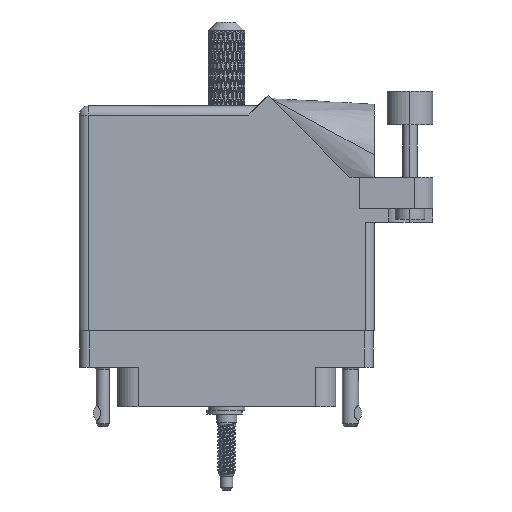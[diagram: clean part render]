
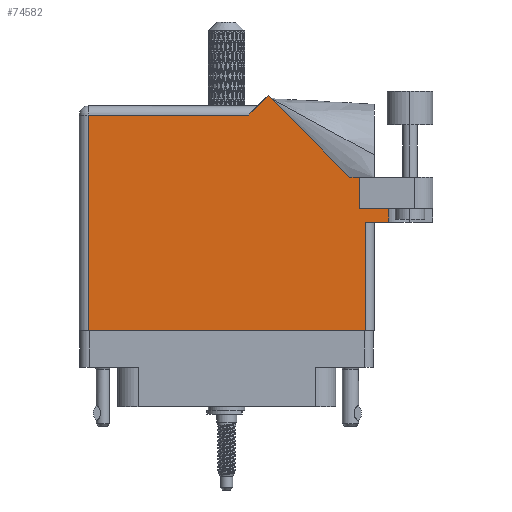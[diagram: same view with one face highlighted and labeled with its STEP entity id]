
A CAD part, front view. The second image highlights one B-rep face of the part: STEP entity #74582.
In plain terms, the highlighted face is planar.
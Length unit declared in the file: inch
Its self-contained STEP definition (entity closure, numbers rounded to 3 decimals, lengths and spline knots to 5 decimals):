
#1 = EDGE_CURVE ( 'NONE', #53166, #113590, #97272, .T. ) ;
#369 = CARTESIAN_POINT ( 'NONE',  ( 0.905, 0.731, 0.455 ) ) ;
#578 = VECTOR ( 'NONE', #109654, 39.37008 ) ;
#999 = DIRECTION ( 'NONE',  ( 0., 1., 0. ) ) ;
#2737 = CARTESIAN_POINT ( 'NONE',  ( 1.1065, 0.731, 0.455 ) ) ;
#3394 = LINE ( 'NONE', #39011, #578 ) ;
#3541 = LINE ( 'NONE', #39164, #83683 ) ;
#3956 = EDGE_CURVE ( 'NONE', #85927, #49844, #56645, .T. ) ;
#6046 = CARTESIAN_POINT ( 'NONE',  ( -1.005, -0.1, 0.455 ) ) ;
#6204 = CARTESIAN_POINT ( 'NONE',  ( 0.83942, 0.944, 0.455 ) ) ;
#7031 = AXIS2_PLACEMENT_3D ( 'NONE', #8806, #87037, #43816 ) ;
#7474 = CARTESIAN_POINT ( 'NONE',  ( -0.943, 1.368, 0.455 ) ) ;
#7632 = CARTESIAN_POINT ( 'NONE',  ( 1.005, 0.637, 0.455 ) ) ;
#8308 = VECTOR ( 'NONE', #999, 39.37008 ) ;
#8493 = DIRECTION ( 'NONE',  ( 0., -1., 0. ) ) ;
#8806 = CARTESIAN_POINT ( 'NONE',  ( -1.005, 1.43, 0.455 ) ) ;
#9829 = CARTESIAN_POINT ( 'NONE',  ( 0.943, -0.1, 0.455 ) ) ;
#13286 = VECTOR ( 'NONE', #91300, 39.37008 ) ;
#14071 = VECTOR ( 'NONE', #58591, 39.37008 ) ;
#14183 = VERTEX_POINT ( 'NONE', #82606 ) ;
#14807 = ORIENTED_EDGE ( 'NONE', *, *, #91940, .T. ) ;
#15362 = VECTOR ( 'NONE', #75333, 39.37008 ) ;
#15830 = CARTESIAN_POINT ( 'NONE',  ( 0.212, 1.43, 0.455 ) ) ;
#16386 = ORIENTED_EDGE ( 'NONE', *, *, #100839, .T. ) ;
#16404 = DIRECTION ( 'NONE',  ( 1., 0., 0. ) ) ;
#17437 = EDGE_CURVE ( 'NONE', #114909, #61215, #83962, .T. ) ;
#17561 = EDGE_CURVE ( 'NONE', #102796, #46006, #89726, .T. ) ;
#19281 = CARTESIAN_POINT ( 'NONE',  ( -0.943, -0.1, 0.455 ) ) ;
#19576 = VECTOR ( 'NONE', #97312, 39.37008 ) ;
#21513 = EDGE_CURVE ( 'NONE', #14183, #114909, #24035, .T. ) ;
#21613 = EDGE_CURVE ( 'NONE', #46006, #49844, #112140, .T. ) ;
#22204 = CARTESIAN_POINT ( 'NONE',  ( 1.1065, 0.637, 0.455 ) ) ;
#22647 = EDGE_LOOP ( 'NONE', ( #14807, #31065, #72263, #29674, #115174, #87179, #88531, #94896, #50619, #61466, #16386 ) ) ;
#24035 = LINE ( 'NONE', #15830, #112729 ) ;
#26243 = EDGE_CURVE ( 'NONE', #53166, #85927, #3394, .T. ) ;
#29674 = ORIENTED_EDGE ( 'NONE', *, *, #3956, .F. ) ;
#31065 = ORIENTED_EDGE ( 'NONE', *, *, #17561, .T. ) ;
#33336 = FACE_OUTER_BOUND ( 'NONE', #22647, .T. ) ;
#36891 = DIRECTION ( 'NONE',  ( -0.707, 0.707, 0. ) ) ;
#39011 = CARTESIAN_POINT ( 'NONE',  ( 0.905, 0.731, 0.455 ) ) ;
#39164 = CARTESIAN_POINT ( 'NONE',  ( 0.83942, 0.944, 0.455 ) ) ;
#41187 = CARTESIAN_POINT ( 'NONE',  ( -0.943, -0.1, 0.455 ) ) ;
#41497 = EDGE_CURVE ( 'NONE', #113590, #89920, #48071, .T. ) ;
#43816 = DIRECTION ( 'NONE',  ( -1., 0., 0. ) ) ;
#45587 = VECTOR ( 'NONE', #8493, 39.37008 ) ;
#46006 = VERTEX_POINT ( 'NONE', #47989 ) ;
#46744 = CARTESIAN_POINT ( 'NONE',  ( 1.1065, 1.06177, 0.455 ) ) ;
#47989 = CARTESIAN_POINT ( 'NONE',  ( 0.943, 0.637, 0.455 ) ) ;
#48071 = LINE ( 'NONE', #93002, #13286 ) ;
#48571 = CARTESIAN_POINT ( 'NONE',  ( 0.905, 0.731, 0.455 ) ) ;
#49844 = VERTEX_POINT ( 'NONE', #22204 ) ;
#50404 = LINE ( 'NONE', #6046, #14071 ) ;
#50619 = ORIENTED_EDGE ( 'NONE', *, *, #21513, .T. ) ;
#53166 = VERTEX_POINT ( 'NONE', #48571 ) ;
#55961 = CARTESIAN_POINT ( 'NONE',  ( 0.15, 1.368, 0.455 ) ) ;
#56645 = LINE ( 'NONE', #46744, #15362 ) ;
#58591 = DIRECTION ( 'NONE',  ( 1., 0., 0. ) ) ;
#60963 = VERTEX_POINT ( 'NONE', #19281 ) ;
#61215 = VERTEX_POINT ( 'NONE', #7474 ) ;
#61466 = ORIENTED_EDGE ( 'NONE', *, *, #17437, .T. ) ;
#62261 = DIRECTION ( 'NONE',  ( 0., 1., 0. ) ) ;
#70109 = DIRECTION ( 'NONE',  ( -0.707, -0.707, 0. ) ) ;
#72263 = ORIENTED_EDGE ( 'NONE', *, *, #21613, .T. ) ;
#74582 = ADVANCED_FACE ( 'NONE', ( #33336 ), #79459, .F. ) ;
#75333 = DIRECTION ( 'NONE',  ( 0., -1., 0. ) ) ;
#76149 = EDGE_CURVE ( 'NONE', #89920, #14183, #3541, .T. ) ;
#78667 = CARTESIAN_POINT ( 'NONE',  ( -1.005, 1.368, 0.455 ) ) ;
#79459 = PLANE ( 'NONE',  #7031 ) ;
#82606 = CARTESIAN_POINT ( 'NONE',  ( 0.28271, 1.50071, 0.455 ) ) ;
#83683 = VECTOR ( 'NONE', #36891, 39.37008 ) ;
#83962 = LINE ( 'NONE', #78667, #19576 ) ;
#85563 = LINE ( 'NONE', #41187, #45587 ) ;
#85927 = VERTEX_POINT ( 'NONE', #2737 ) ;
#87037 = DIRECTION ( 'NONE',  ( 0., 0., -1. ) ) ;
#87179 = ORIENTED_EDGE ( 'NONE', *, *, #1, .T. ) ;
#88531 = ORIENTED_EDGE ( 'NONE', *, *, #41497, .T. ) ;
#89726 = LINE ( 'NONE', #92449, #8308 ) ;
#89920 = VERTEX_POINT ( 'NONE', #6204 ) ;
#91300 = DIRECTION ( 'NONE',  ( -1., 0., 0. ) ) ;
#91940 = EDGE_CURVE ( 'NONE', #60963, #102796, #50404, .T. ) ;
#92241 = VECTOR ( 'NONE', #16404, 39.37008 ) ;
#92449 = CARTESIAN_POINT ( 'NONE',  ( 0.943, 0.637, 0.455 ) ) ;
#93002 = CARTESIAN_POINT ( 'NONE',  ( 1.405, 0.944, 0.455 ) ) ;
#94896 = ORIENTED_EDGE ( 'NONE', *, *, #76149, .T. ) ;
#97018 = VECTOR ( 'NONE', #62261, 39.37008 ) ;
#97272 = LINE ( 'NONE', #369, #97018 ) ;
#97312 = DIRECTION ( 'NONE',  ( -1., 0., 0. ) ) ;
#100839 = EDGE_CURVE ( 'NONE', #61215, #60963, #85563, .T. ) ;
#102796 = VERTEX_POINT ( 'NONE', #9829 ) ;
#109654 = DIRECTION ( 'NONE',  ( 1., 0., 0. ) ) ;
#110814 = CARTESIAN_POINT ( 'NONE',  ( 0.905, 0.944, 0.455 ) ) ;
#112140 = LINE ( 'NONE', #7632, #92241 ) ;
#112729 = VECTOR ( 'NONE', #70109, 39.37008 ) ;
#113590 = VERTEX_POINT ( 'NONE', #110814 ) ;
#114909 = VERTEX_POINT ( 'NONE', #55961 ) ;
#115174 = ORIENTED_EDGE ( 'NONE', *, *, #26243, .F. ) ;
